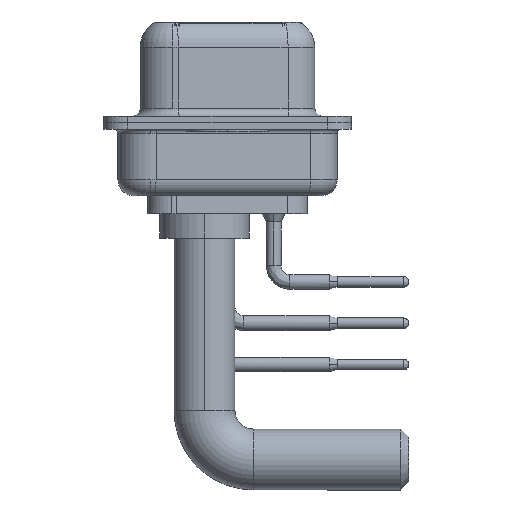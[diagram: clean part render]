
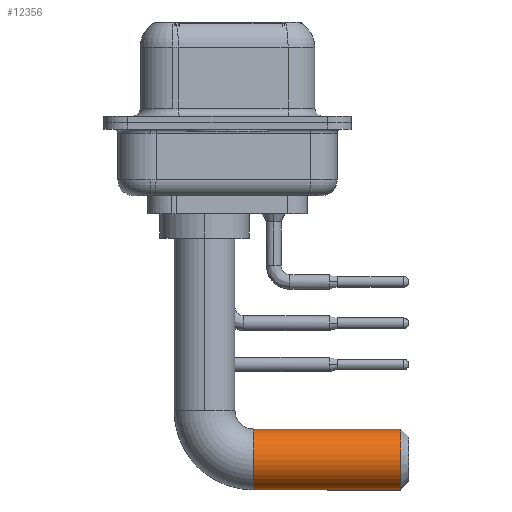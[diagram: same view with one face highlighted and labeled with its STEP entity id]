
A CAD part, left-side view. The second image highlights one B-rep face of the part: STEP entity #12356.
In plain terms, the highlighted cylindrical face has radius 1.875 mm (diameter 3.75 mm), a partial arc.
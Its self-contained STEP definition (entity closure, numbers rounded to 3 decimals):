
#123 = EDGE_LOOP ( 'NONE', ( #16158, #21020, #20354, #9701 ) ) ;
#1477 = CIRCLE ( 'NONE', #24825, 1.875 ) ;
#1995 = VERTEX_POINT ( 'NONE', #23455 ) ;
#2494 = CARTESIAN_POINT ( 'NONE',  ( 0., -12.07, -15.505 ) ) ;
#2842 = CYLINDRICAL_SURFACE ( 'NONE', #8818, 1.875 ) ;
#3557 = DIRECTION ( 'NONE',  ( 0., 1., 0. ) ) ;
#3964 = CARTESIAN_POINT ( 'NONE',  ( 0., -12.07, -11.755 ) ) ;
#6461 = DIRECTION ( 'NONE',  ( 0., -1., 0. ) ) ;
#7112 = VERTEX_POINT ( 'NONE', #3964 ) ;
#7865 = DIRECTION ( 'NONE',  ( 0., -1., 0. ) ) ;
#8818 = AXIS2_PLACEMENT_3D ( 'NONE', #12737, #7865, #17789 ) ;
#9701 = ORIENTED_EDGE ( 'NONE', *, *, #20320, .T. ) ;
#9785 = EDGE_CURVE ( 'NONE', #28513, #7112, #31340, .T. ) ;
#10205 = EDGE_CURVE ( 'NONE', #28513, #1995, #13957, .T. ) ;
#10623 = FACE_OUTER_BOUND ( 'NONE', #123, .T. ) ;
#11014 = DIRECTION ( 'NONE',  ( 0., 0., -1. ) ) ;
#11491 = VECTOR ( 'NONE', #6461, 1000. ) ;
#12356 = ADVANCED_FACE ( 'NONE', ( #10623 ), #2842, .T. ) ;
#12737 = CARTESIAN_POINT ( 'NONE',  ( 0., -3., -13.63 ) ) ;
#13216 = CARTESIAN_POINT ( 'NONE',  ( 0., -3., -15.505 ) ) ;
#13957 = CIRCLE ( 'NONE', #31123, 1.875 ) ;
#15777 = VECTOR ( 'NONE', #19035, 1000. ) ;
#16158 = ORIENTED_EDGE ( 'NONE', *, *, #9785, .F. ) ;
#17789 = DIRECTION ( 'NONE',  ( 0., 0., -1. ) ) ;
#19003 = DIRECTION ( 'NONE',  ( -1., 0., 0. ) ) ;
#19035 = DIRECTION ( 'NONE',  ( 0., -1., 0. ) ) ;
#20320 = EDGE_CURVE ( 'NONE', #30282, #7112, #1477, .T. ) ;
#20354 = ORIENTED_EDGE ( 'NONE', *, *, #26745, .T. ) ;
#21020 = ORIENTED_EDGE ( 'NONE', *, *, #10205, .T. ) ;
#21459 = LINE ( 'NONE', #13216, #15777 ) ;
#23455 = CARTESIAN_POINT ( 'NONE',  ( 0., -3., -15.505 ) ) ;
#23883 = CARTESIAN_POINT ( 'NONE',  ( 0., -3., -13.63 ) ) ;
#24825 = AXIS2_PLACEMENT_3D ( 'NONE', #28607, #3557, #11014 ) ;
#26745 = EDGE_CURVE ( 'NONE', #1995, #30282, #21459, .T. ) ;
#27737 = CARTESIAN_POINT ( 'NONE',  ( 0., -3., -11.755 ) ) ;
#28513 = VERTEX_POINT ( 'NONE', #27737 ) ;
#28607 = CARTESIAN_POINT ( 'NONE',  ( 0., -12.07, -13.63 ) ) ;
#30282 = VERTEX_POINT ( 'NONE', #2494 ) ;
#31016 = CARTESIAN_POINT ( 'NONE',  ( 0., -3., -11.755 ) ) ;
#31123 = AXIS2_PLACEMENT_3D ( 'NONE', #23883, #31531, #19003 ) ;
#31340 = LINE ( 'NONE', #31016, #11491 ) ;
#31531 = DIRECTION ( 'NONE',  ( 0., -1., 0. ) ) ;
